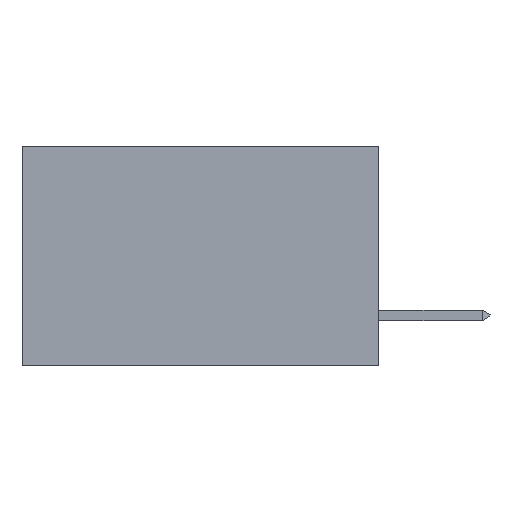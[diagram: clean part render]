
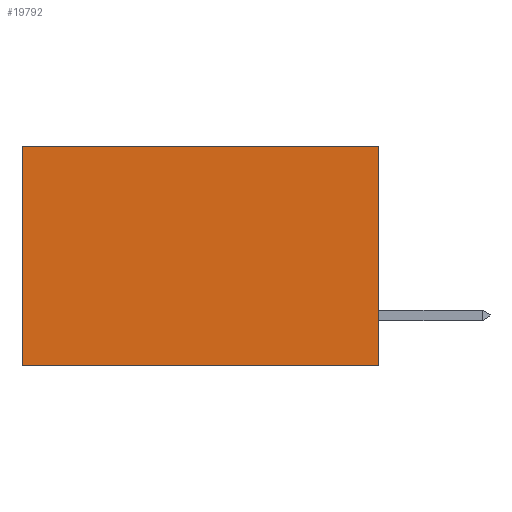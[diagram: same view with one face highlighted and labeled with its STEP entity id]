
A CAD part, left-side view. The second image highlights one B-rep face of the part: STEP entity #19792.
In plain terms, the highlighted planar face has unit normal (-1, 0, 0).
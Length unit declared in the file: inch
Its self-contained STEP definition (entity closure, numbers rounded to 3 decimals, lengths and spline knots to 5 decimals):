
#2 = CARTESIAN_POINT ( 'NONE',  ( 0.298, 0.6, 0. ) ) ;
#882 = DIRECTION ( 'NONE',  ( 0., 1., 0. ) ) ;
#1067 = AXIS2_PLACEMENT_3D ( 'NONE', #1191, #14066, #5964 ) ;
#1191 = CARTESIAN_POINT ( 'NONE',  ( 0.298, 0., 0. ) ) ;
#1583 = CARTESIAN_POINT ( 'NONE',  ( 0.298, 0.6, 0. ) ) ;
#1914 = VECTOR ( 'NONE', #882, 39.37008 ) ;
#2291 = DIRECTION ( 'NONE',  ( 0., 0., -1. ) ) ;
#3547 = CARTESIAN_POINT ( 'NONE',  ( 0.298, 0., -0.37 ) ) ;
#4481 = CARTESIAN_POINT ( 'NONE',  ( 0.298, 0., -0.37 ) ) ;
#4619 = FACE_OUTER_BOUND ( 'NONE', #19927, .T. ) ;
#4913 = VERTEX_POINT ( 'NONE', #13130 ) ;
#5964 = DIRECTION ( 'NONE',  ( 0., 0., -1. ) ) ;
#7667 = PLANE ( 'NONE',  #1067 ) ;
#8754 = VERTEX_POINT ( 'NONE', #1583 ) ;
#9841 = ORIENTED_EDGE ( 'NONE', *, *, #16520, .F. ) ;
#10565 = ORIENTED_EDGE ( 'NONE', *, *, #25313, .T. ) ;
#11087 = LINE ( 'NONE', #11624, #1914 ) ;
#11624 = CARTESIAN_POINT ( 'NONE',  ( 0.298, 0., 0. ) ) ;
#12255 = VECTOR ( 'NONE', #2291, 39.37008 ) ;
#12489 = VERTEX_POINT ( 'NONE', #14798 ) ;
#12896 = DIRECTION ( 'NONE',  ( 0., 0., -1. ) ) ;
#13130 = CARTESIAN_POINT ( 'NONE',  ( 0.298, 0., 0. ) ) ;
#13304 = ORIENTED_EDGE ( 'NONE', *, *, #18119, .T. ) ;
#14066 = DIRECTION ( 'NONE',  ( 1., 0., 0. ) ) ;
#14798 = CARTESIAN_POINT ( 'NONE',  ( 0.298, 0.6, -0.37 ) ) ;
#16450 = LINE ( 'NONE', #21373, #20511 ) ;
#16520 = EDGE_CURVE ( 'NONE', #18912, #12489, #16535, .T. ) ;
#16535 = LINE ( 'NONE', #4481, #21287 ) ;
#17810 = EDGE_CURVE ( 'NONE', #4913, #18912, #16450, .T. ) ;
#18119 = EDGE_CURVE ( 'NONE', #4913, #8754, #11087, .T. ) ;
#18912 = VERTEX_POINT ( 'NONE', #3547 ) ;
#19792 = ADVANCED_FACE ( 'NONE', ( #4619 ), #7667, .F. ) ;
#19927 = EDGE_LOOP ( 'NONE', ( #10565, #9841, #23426, #13304 ) ) ;
#20511 = VECTOR ( 'NONE', #12896, 39.37008 ) ;
#21287 = VECTOR ( 'NONE', #25326, 39.37008 ) ;
#21373 = CARTESIAN_POINT ( 'NONE',  ( 0.298, 0., 0. ) ) ;
#23335 = LINE ( 'NONE', #2, #12255 ) ;
#23426 = ORIENTED_EDGE ( 'NONE', *, *, #17810, .F. ) ;
#25313 = EDGE_CURVE ( 'NONE', #8754, #12489, #23335, .T. ) ;
#25326 = DIRECTION ( 'NONE',  ( 0., 1., 0. ) ) ;
